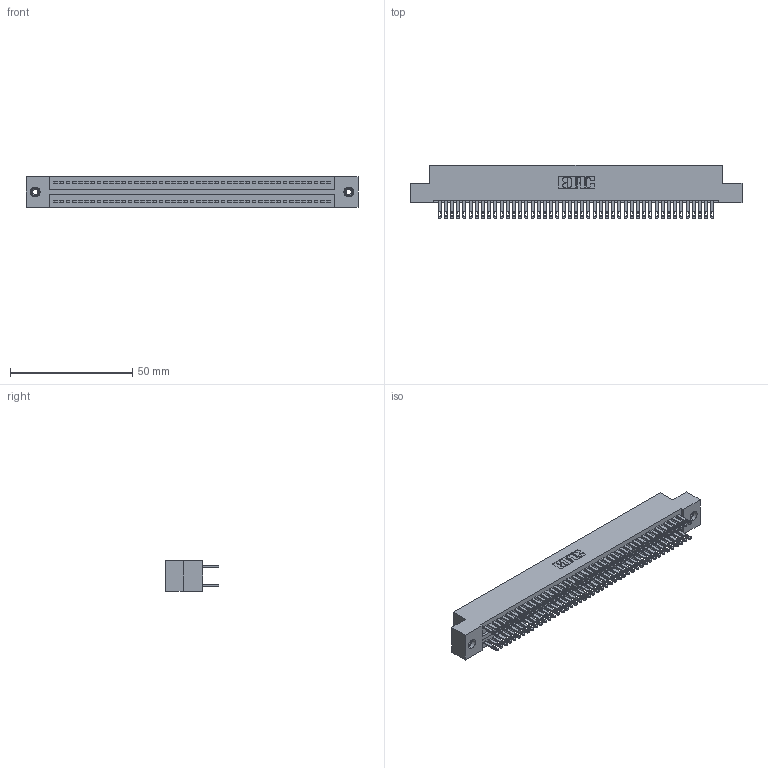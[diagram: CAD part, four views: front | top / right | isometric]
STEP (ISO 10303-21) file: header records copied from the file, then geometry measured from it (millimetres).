
FILE_DESCRIPTION (( 'STEP AP203' ), '1' );
FILE_NAME ('325-090-500-208.STEP', '2020-02-25T05:34:37', ( '' ), ( '' ), 'SwSTEP 2.0', 'SolidWorks 2016', '' );
FILE_SCHEMA (( 'CONFIG_CONTROL_DESIGN' ));
Length unit declared in the file: inch
Products named in the file (4): 325-090-500-208; 325-292-001_325-293-100; 325 Part_TI; 345-250-001_345-250-003-102
Assembly tree (93 placements, depth 2):
  325-090-500-208
    325 Part_TI
    325-292-001_325-293-100  x90
    345-250-001_345-250-003-102  x2
Bounding box: 136.02 x 21.84 x 12.45 mm (x, y, z)
Volume: 17854.6 mm3; surface area: 22636.5 mm2
Topology: 93 solids, 93 shells, 4494 faces, 13677 edges, 9110 vertices
Faces by surface type: plane 2802, cylinder 1676, cone 12, torus 4
Entity records: 29678 total; most frequent: CARTESIAN_POINT 4897, ORIENTED_EDGE 4826, DIRECTION 4211, EDGE_CURVE 2413, VECTOR 2261, LINE 2261, VERTEX_POINT 1604, AXIS2_PLACEMENT_3D 975
